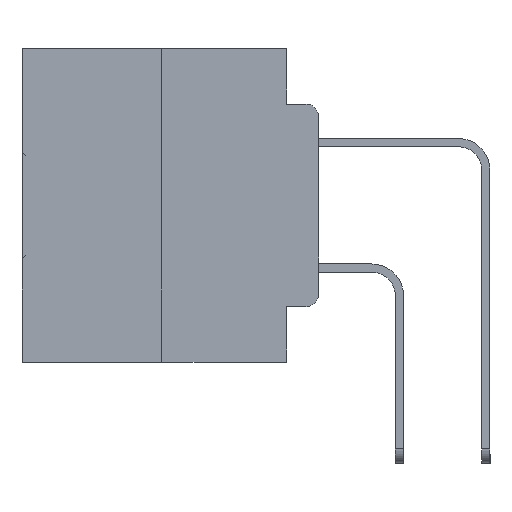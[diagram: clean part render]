
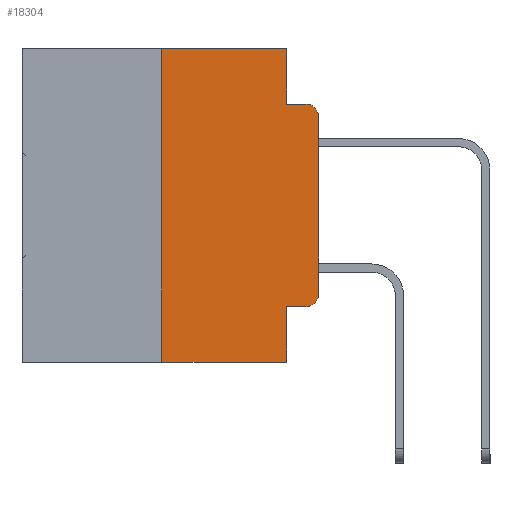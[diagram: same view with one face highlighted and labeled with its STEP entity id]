
A CAD part, left-side view. The second image highlights one B-rep face of the part: STEP entity #18304.
In plain terms, the highlighted planar face has unit normal (-1, 0, 0).
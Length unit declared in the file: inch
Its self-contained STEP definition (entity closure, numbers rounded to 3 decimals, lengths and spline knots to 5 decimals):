
#222 = VECTOR ( 'NONE', #3564, 39.37008 ) ;
#686 = CIRCLE ( 'NONE', #16711, 0.02 ) ;
#1802 = ORIENTED_EDGE ( 'NONE', *, *, #33913, .T. ) ;
#2092 = CARTESIAN_POINT ( 'NONE',  ( 0., 0.25, -0.5 ) ) ;
#2792 = ORIENTED_EDGE ( 'NONE', *, *, #26158, .T. ) ;
#3564 = DIRECTION ( 'NONE',  ( 0., -1., 0. ) ) ;
#3740 = VECTOR ( 'NONE', #7668, 39.37008 ) ;
#3987 = CIRCLE ( 'NONE', #20963, 0.02 ) ;
#4043 = ORIENTED_EDGE ( 'NONE', *, *, #16889, .T. ) ;
#4063 = LINE ( 'NONE', #15816, #17520 ) ;
#4591 = LINE ( 'NONE', #31962, #3740 ) ;
#4678 = VERTEX_POINT ( 'NONE', #30406 ) ;
#4935 = DIRECTION ( 'NONE',  ( 0., 0., -1. ) ) ;
#5205 = ORIENTED_EDGE ( 'NONE', *, *, #27108, .F. ) ;
#5433 = CARTESIAN_POINT ( 'NONE',  ( 0., 0., -0.1085 ) ) ;
#6008 = ORIENTED_EDGE ( 'NONE', *, *, #13669, .F. ) ;
#6380 = CARTESIAN_POINT ( 'NONE',  ( 0., 0.051, -0.4115 ) ) ;
#7513 = PLANE ( 'NONE',  #9517 ) ;
#7668 = DIRECTION ( 'NONE',  ( 0., -1., 0. ) ) ;
#8302 = VECTOR ( 'NONE', #33759, 39.37008 ) ;
#9021 = VERTEX_POINT ( 'NONE', #2092 ) ;
#9517 = AXIS2_PLACEMENT_3D ( 'NONE', #29247, #21114, #4935 ) ;
#12330 = DIRECTION ( 'NONE',  ( -1., 0., 0. ) ) ;
#12757 = CARTESIAN_POINT ( 'NONE',  ( 0., 0.02, -0.3915 ) ) ;
#13669 = EDGE_CURVE ( 'NONE', #17683, #21093, #15461, .T. ) ;
#13855 = VECTOR ( 'NONE', #30493, 39.37008 ) ;
#14168 = CARTESIAN_POINT ( 'NONE',  ( 0., 0.051, 0. ) ) ;
#14229 = CARTESIAN_POINT ( 'NONE',  ( 0., 0.25, 0. ) ) ;
#14530 = LINE ( 'NONE', #27867, #222 ) ;
#14937 = DIRECTION ( 'NONE',  ( 0., -1., 0. ) ) ;
#15451 = DIRECTION ( 'NONE',  ( 0., 0., -1. ) ) ;
#15461 = LINE ( 'NONE', #31106, #8302 ) ;
#15752 = FACE_OUTER_BOUND ( 'NONE', #24644, .T. ) ;
#15816 = CARTESIAN_POINT ( 'NONE',  ( 0., 0., 0. ) ) ;
#16047 = ORIENTED_EDGE ( 'NONE', *, *, #31939, .T. ) ;
#16521 = VERTEX_POINT ( 'NONE', #26212 ) ;
#16711 = AXIS2_PLACEMENT_3D ( 'NONE', #12757, #31756, #15451 ) ;
#16889 = EDGE_CURVE ( 'NONE', #19274, #17272, #14530, .T. ) ;
#17272 = VERTEX_POINT ( 'NONE', #29379 ) ;
#17520 = VECTOR ( 'NONE', #18586, 39.37008 ) ;
#17683 = VERTEX_POINT ( 'NONE', #21281 ) ;
#17951 = ORIENTED_EDGE ( 'NONE', *, *, #29536, .F. ) ;
#17958 = EDGE_CURVE ( 'NONE', #9021, #17683, #32730, .T. ) ;
#18304 = ADVANCED_FACE ( 'NONE', ( #15752 ), #7513, .F. ) ;
#18586 = DIRECTION ( 'NONE',  ( 0., 0., 1. ) ) ;
#18680 = DIRECTION ( 'NONE',  ( 0., 0., -1. ) ) ;
#18770 = LINE ( 'NONE', #29663, #26919 ) ;
#19274 = VERTEX_POINT ( 'NONE', #6380 ) ;
#19680 = EDGE_CURVE ( 'NONE', #19274, #22424, #28370, .T. ) ;
#20295 = VECTOR ( 'NONE', #14937, 39.37008 ) ;
#20514 = CARTESIAN_POINT ( 'NONE',  ( 0., 0.051, 0. ) ) ;
#20963 = AXIS2_PLACEMENT_3D ( 'NONE', #28645, #12330, #31334 ) ;
#21093 = VERTEX_POINT ( 'NONE', #20514 ) ;
#21114 = DIRECTION ( 'NONE',  ( 1., 0., 0. ) ) ;
#21281 = CARTESIAN_POINT ( 'NONE',  ( 0., 0.25, 0. ) ) ;
#22424 = VERTEX_POINT ( 'NONE', #24066 ) ;
#22491 = VERTEX_POINT ( 'NONE', #5433 ) ;
#23825 = ORIENTED_EDGE ( 'NONE', *, *, #26487, .T. ) ;
#24066 = CARTESIAN_POINT ( 'NONE',  ( 0., 0.051, -0.5 ) ) ;
#24644 = EDGE_LOOP ( 'NONE', ( #23825, #16047, #17951, #5205, #6008, #25920, #1802, #33203, #4043, #2792 ) ) ;
#25920 = ORIENTED_EDGE ( 'NONE', *, *, #17958, .F. ) ;
#26158 = EDGE_CURVE ( 'NONE', #17272, #16521, #686, .T. ) ;
#26212 = CARTESIAN_POINT ( 'NONE',  ( 0., 0., -0.3915 ) ) ;
#26436 = VECTOR ( 'NONE', #30554, 39.37008 ) ;
#26487 = EDGE_CURVE ( 'NONE', #16521, #22491, #4063, .T. ) ;
#26919 = VECTOR ( 'NONE', #18680, 39.37008 ) ;
#27108 = EDGE_CURVE ( 'NONE', #21093, #4678, #18770, .T. ) ;
#27867 = CARTESIAN_POINT ( 'NONE',  ( 0., 0.051, -0.4115 ) ) ;
#28370 = LINE ( 'NONE', #14168, #13855 ) ;
#28645 = CARTESIAN_POINT ( 'NONE',  ( 0., 0.02, -0.1085 ) ) ;
#29247 = CARTESIAN_POINT ( 'NONE',  ( 0., 0.473, 0. ) ) ;
#29379 = CARTESIAN_POINT ( 'NONE',  ( 0., 0.02, -0.4115 ) ) ;
#29536 = EDGE_CURVE ( 'NONE', #4678, #34273, #4591, .T. ) ;
#29663 = CARTESIAN_POINT ( 'NONE',  ( 0., 0.051, 0. ) ) ;
#30406 = CARTESIAN_POINT ( 'NONE',  ( 0., 0.051, -0.0885 ) ) ;
#30493 = DIRECTION ( 'NONE',  ( 0., 0., -1. ) ) ;
#30554 = DIRECTION ( 'NONE',  ( 0., 0., 1. ) ) ;
#31106 = CARTESIAN_POINT ( 'NONE',  ( 0., 0.473, 0. ) ) ;
#31248 = CARTESIAN_POINT ( 'NONE',  ( 0., 0.473, -0.5 ) ) ;
#31334 = DIRECTION ( 'NONE',  ( 0., 0., -1. ) ) ;
#31756 = DIRECTION ( 'NONE',  ( -1., 0., 0. ) ) ;
#31939 = EDGE_CURVE ( 'NONE', #22491, #34273, #3987, .T. ) ;
#31962 = CARTESIAN_POINT ( 'NONE',  ( 0., 0.051, -0.0885 ) ) ;
#32730 = LINE ( 'NONE', #14229, #26436 ) ;
#32737 = CARTESIAN_POINT ( 'NONE',  ( 0., 0.02, -0.0885 ) ) ;
#33203 = ORIENTED_EDGE ( 'NONE', *, *, #19680, .F. ) ;
#33759 = DIRECTION ( 'NONE',  ( 0., -1., 0. ) ) ;
#33913 = EDGE_CURVE ( 'NONE', #9021, #22424, #34683, .T. ) ;
#34273 = VERTEX_POINT ( 'NONE', #32737 ) ;
#34683 = LINE ( 'NONE', #31248, #20295 ) ;
